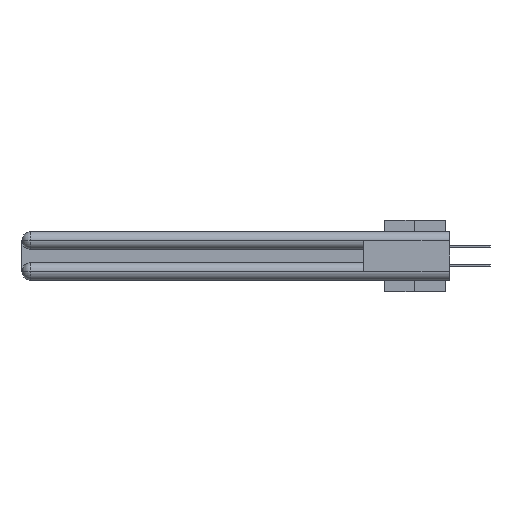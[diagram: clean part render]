
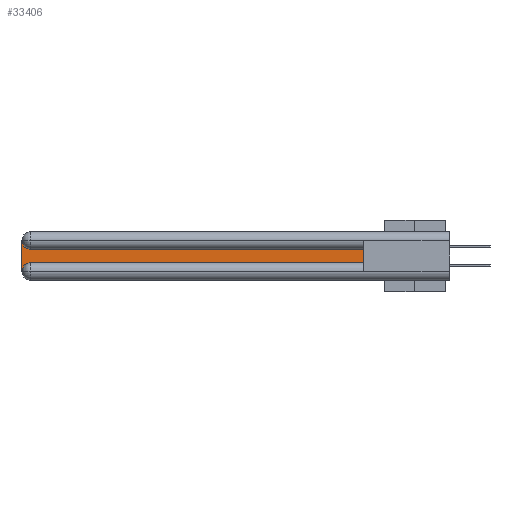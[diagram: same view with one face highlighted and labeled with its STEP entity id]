
A CAD part, left-side view. The second image highlights one B-rep face of the part: STEP entity #33406.
In plain terms, the highlighted planar face has unit normal (-1, 0, 0).
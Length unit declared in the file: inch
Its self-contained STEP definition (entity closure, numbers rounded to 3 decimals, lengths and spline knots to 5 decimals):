
#213 = DIRECTION ( 'NONE',  ( 0., 1., 0. ) ) ;
#1252 = VERTEX_POINT ( 'NONE', #24094 ) ;
#3237 = ORIENTED_EDGE ( 'NONE', *, *, #43322, .T. ) ;
#4864 = VECTOR ( 'NONE', #21654, 39.37008 ) ;
#6873 = DIRECTION ( 'NONE',  ( 1., 0., 0. ) ) ;
#6882 = EDGE_CURVE ( 'NONE', #11765, #1252, #38890, .T. ) ;
#7517 = DIRECTION ( 'NONE',  ( 0., 0., -1. ) ) ;
#7871 = ORIENTED_EDGE ( 'NONE', *, *, #6882, .T. ) ;
#7980 = DIRECTION ( 'NONE',  ( 0., -1., 0. ) ) ;
#10390 = CARTESIAN_POINT ( 'NONE',  ( 0.075, 2.94, -0.1225 ) ) ;
#10486 = DIRECTION ( 'NONE',  ( 0., 0., -1. ) ) ;
#11765 = VERTEX_POINT ( 'NONE', #48427 ) ;
#12135 = ORIENTED_EDGE ( 'NONE', *, *, #35349, .T. ) ;
#13539 = VERTEX_POINT ( 'NONE', #29265 ) ;
#13949 = LINE ( 'NONE', #29059, #31703 ) ;
#15309 = CARTESIAN_POINT ( 'NONE',  ( 0.075, 0.6, -0.1225 ) ) ;
#16796 = CARTESIAN_POINT ( 'NONE',  ( 0.075, 3., -0.1225 ) ) ;
#20332 = CIRCLE ( 'NONE', #24925, 0.06 ) ;
#21654 = DIRECTION ( 'NONE',  ( 0., 0., 1. ) ) ;
#21816 = ORIENTED_EDGE ( 'NONE', *, *, #37483, .T. ) ;
#22508 = CARTESIAN_POINT ( 'NONE',  ( 0.075, 3., -0.0625 ) ) ;
#24094 = CARTESIAN_POINT ( 'NONE',  ( 0.075, 0.6, -0.2175 ) ) ;
#24486 = VERTEX_POINT ( 'NONE', #41354 ) ;
#24925 = AXIS2_PLACEMENT_3D ( 'NONE', #41316, #6873, #45151 ) ;
#25827 = ORIENTED_EDGE ( 'NONE', *, *, #48039, .T. ) ;
#27439 = LINE ( 'NONE', #47768, #4864 ) ;
#27558 = DIRECTION ( 'NONE',  ( 1., 0., 0. ) ) ;
#28050 = DIRECTION ( 'NONE',  ( 0., 0., -1. ) ) ;
#28526 = VECTOR ( 'NONE', #213, 39.37008 ) ;
#29059 = CARTESIAN_POINT ( 'NONE',  ( 0.075, 3., -0.2175 ) ) ;
#29265 = CARTESIAN_POINT ( 'NONE',  ( 0.075, 3., -0.2775 ) ) ;
#29581 = FACE_OUTER_BOUND ( 'NONE', #48670, .T. ) ;
#29893 = CARTESIAN_POINT ( 'NONE',  ( 0.075, 2.94, -0.2775 ) ) ;
#30090 = EDGE_CURVE ( 'NONE', #13539, #11765, #32143, .T. ) ;
#31411 = AXIS2_PLACEMENT_3D ( 'NONE', #29893, #41628, #7517 ) ;
#31485 = PLANE ( 'NONE',  #32147 ) ;
#31703 = VECTOR ( 'NONE', #10486, 39.37008 ) ;
#31811 = CARTESIAN_POINT ( 'NONE',  ( 0.075, 0.6, -0.2175 ) ) ;
#32143 = CIRCLE ( 'NONE', #31411, 0.06 ) ;
#32147 = AXIS2_PLACEMENT_3D ( 'NONE', #16796, #27558, #28050 ) ;
#33406 = ADVANCED_FACE ( 'NONE', ( #29581 ), #31485, .F. ) ;
#35349 = EDGE_CURVE ( 'NONE', #41599, #13539, #13949, .T. ) ;
#37483 = EDGE_CURVE ( 'NONE', #24486, #42703, #47457, .T. ) ;
#38890 = LINE ( 'NONE', #31811, #43018 ) ;
#41316 = CARTESIAN_POINT ( 'NONE',  ( 0.075, 2.94, -0.0625 ) ) ;
#41354 = CARTESIAN_POINT ( 'NONE',  ( 0.075, 0.6, -0.1225 ) ) ;
#41599 = VERTEX_POINT ( 'NONE', #22508 ) ;
#41628 = DIRECTION ( 'NONE',  ( 1., 0., 0. ) ) ;
#41908 = ORIENTED_EDGE ( 'NONE', *, *, #30090, .T. ) ;
#42703 = VERTEX_POINT ( 'NONE', #10390 ) ;
#43018 = VECTOR ( 'NONE', #7980, 39.37008 ) ;
#43322 = EDGE_CURVE ( 'NONE', #42703, #41599, #20332, .T. ) ;
#45151 = DIRECTION ( 'NONE',  ( 0., 0., -1. ) ) ;
#47457 = LINE ( 'NONE', #15309, #28526 ) ;
#47768 = CARTESIAN_POINT ( 'NONE',  ( 0.075, 0.6, -0.2175 ) ) ;
#48039 = EDGE_CURVE ( 'NONE', #1252, #24486, #27439, .T. ) ;
#48427 = CARTESIAN_POINT ( 'NONE',  ( 0.075, 2.94, -0.2175 ) ) ;
#48670 = EDGE_LOOP ( 'NONE', ( #21816, #3237, #12135, #41908, #7871, #25827 ) ) ;
